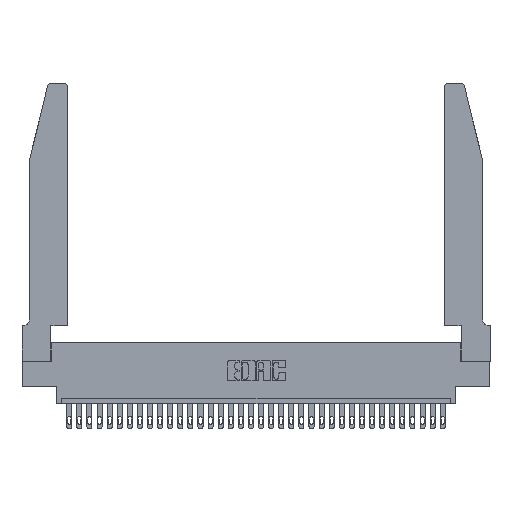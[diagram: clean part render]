
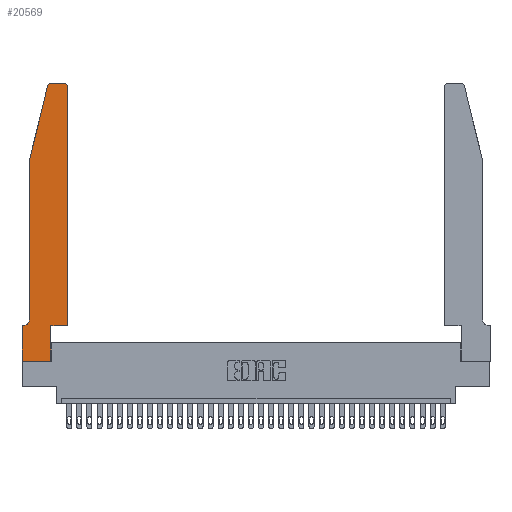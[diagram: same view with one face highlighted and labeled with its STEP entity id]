
A CAD part, top view. The second image highlights one B-rep face of the part: STEP entity #20569.
In plain terms, the highlighted planar face has unit normal (0, 0, 1).
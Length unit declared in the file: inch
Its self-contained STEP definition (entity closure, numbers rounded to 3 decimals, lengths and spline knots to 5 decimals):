
#305 = EDGE_CURVE ( 'NONE', #24303, #15757, #10780, .T. ) ;
#506 = CARTESIAN_POINT ( 'NONE',  ( 0.284, 2.72, 0.37 ) ) ;
#905 = CARTESIAN_POINT ( 'NONE',  ( 0.284, 2.75, 0.37 ) ) ;
#1224 = DIRECTION ( 'NONE',  ( 0., -1., 0. ) ) ;
#1340 = DIRECTION ( 'NONE',  ( 0., 0., -1. ) ) ;
#1395 = CARTESIAN_POINT ( 'NONE',  ( 0.4505, 2.72, 0.37 ) ) ;
#1404 = EDGE_CURVE ( 'NONE', #18840, #24303, #11525, .T. ) ;
#1493 = DIRECTION ( 'NONE',  ( -1., 0., 0. ) ) ;
#2607 = CARTESIAN_POINT ( 'NONE',  ( 0.4505, 0.35, 0.37 ) ) ;
#3799 = CARTESIAN_POINT ( 'NONE',  ( 0.4505, 0.35, 0.37 ) ) ;
#4000 = AXIS2_PLACEMENT_3D ( 'NONE', #31389, #18379, #26298 ) ;
#4079 = CARTESIAN_POINT ( 'NONE',  ( 0.4205, 2.75, 0.37 ) ) ;
#4186 = VERTEX_POINT ( 'NONE', #13802 ) ;
#4364 = VECTOR ( 'NONE', #33023, 39.37008 ) ;
#4469 = DIRECTION ( 'NONE',  ( 0., 0., 1. ) ) ;
#4846 = ORIENTED_EDGE ( 'NONE', *, *, #305, .T. ) ;
#4898 = VERTEX_POINT ( 'NONE', #23173 ) ;
#6002 = LINE ( 'NONE', #12059, #4364 ) ;
#6209 = CARTESIAN_POINT ( 'NONE',  ( 0.0755, 2., 0.37 ) ) ;
#6503 = LINE ( 'NONE', #12912, #21293 ) ;
#6768 = AXIS2_PLACEMENT_3D ( 'NONE', #17892, #4469, #20534 ) ;
#7193 = ORIENTED_EDGE ( 'NONE', *, *, #22379, .T. ) ;
#7827 = CARTESIAN_POINT ( 'NONE',  ( 0.0755, 0.35, 0.37 ) ) ;
#7880 = VECTOR ( 'NONE', #12998, 39.37008 ) ;
#8034 = ORIENTED_EDGE ( 'NONE', *, *, #8875, .T. ) ;
#8471 = EDGE_CURVE ( 'NONE', #13320, #4898, #28889, .T. ) ;
#8622 = LINE ( 'NONE', #22801, #30417 ) ;
#8875 = EDGE_CURVE ( 'NONE', #31925, #20930, #32997, .T. ) ;
#9761 = CARTESIAN_POINT ( 'NONE',  ( 0.0755, 2., 0.37 ) ) ;
#10780 = LINE ( 'NONE', #9761, #28857 ) ;
#11525 = CIRCLE ( 'NONE', #24944, 0.03 ) ;
#11659 = EDGE_CURVE ( 'NONE', #16005, #18840, #8622, .T. ) ;
#12059 = CARTESIAN_POINT ( 'NONE',  ( 0., 0., 0.37 ) ) ;
#12116 = LINE ( 'NONE', #7827, #25252 ) ;
#12176 = ORIENTED_EDGE ( 'NONE', *, *, #8471, .T. ) ;
#12217 = CARTESIAN_POINT ( 'NONE',  ( 0.0755, 0.42, 0.37 ) ) ;
#12607 = PLANE ( 'NONE',  #6768 ) ;
#12912 = CARTESIAN_POINT ( 'NONE',  ( 0.0755, 2., 0.37 ) ) ;
#12998 = DIRECTION ( 'NONE',  ( 0., 1., 0. ) ) ;
#13320 = VERTEX_POINT ( 'NONE', #28864 ) ;
#13802 = CARTESIAN_POINT ( 'NONE',  ( 0.4505, 0.35, 0.37 ) ) ;
#14091 = VECTOR ( 'NONE', #20321, 39.37008 ) ;
#14521 = VECTOR ( 'NONE', #1224, 39.37008 ) ;
#14833 = LINE ( 'NONE', #3799, #16866 ) ;
#14865 = LINE ( 'NONE', #2607, #7880 ) ;
#14997 = CIRCLE ( 'NONE', #21307, 0.07 ) ;
#15329 = DIRECTION ( 'NONE',  ( 0., -1., 0. ) ) ;
#15757 = VERTEX_POINT ( 'NONE', #6209 ) ;
#16005 = VERTEX_POINT ( 'NONE', #4079 ) ;
#16279 = ORIENTED_EDGE ( 'NONE', *, *, #22177, .T. ) ;
#16815 = VERTEX_POINT ( 'NONE', #12217 ) ;
#16866 = VECTOR ( 'NONE', #29827, 39.37008 ) ;
#17140 = CARTESIAN_POINT ( 'NONE',  ( 0., 0., 0.37 ) ) ;
#17892 = CARTESIAN_POINT ( 'NONE',  ( 0., 0.35, 0.37 ) ) ;
#18133 = ORIENTED_EDGE ( 'NONE', *, *, #30949, .T. ) ;
#18219 = VERTEX_POINT ( 'NONE', #1395 ) ;
#18251 = ORIENTED_EDGE ( 'NONE', *, *, #11659, .T. ) ;
#18259 = CIRCLE ( 'NONE', #4000, 0.03 ) ;
#18379 = DIRECTION ( 'NONE',  ( 0., 0., 1. ) ) ;
#18840 = VERTEX_POINT ( 'NONE', #905 ) ;
#19017 = ORIENTED_EDGE ( 'NONE', *, *, #1404, .T. ) ;
#19186 = DIRECTION ( 'NONE',  ( -1., 0., 0. ) ) ;
#19715 = EDGE_CURVE ( 'NONE', #20930, #13320, #6002, .T. ) ;
#20290 = FACE_OUTER_BOUND ( 'NONE', #28917, .T. ) ;
#20321 = DIRECTION ( 'NONE',  ( 0., 1., 0. ) ) ;
#20534 = DIRECTION ( 'NONE',  ( 1., 0., 0. ) ) ;
#20569 = ADVANCED_FACE ( 'NONE', ( #20290 ), #12607, .T. ) ;
#20879 = ORIENTED_EDGE ( 'NONE', *, *, #32941, .T. ) ;
#20930 = VERTEX_POINT ( 'NONE', #17140 ) ;
#21264 = ORIENTED_EDGE ( 'NONE', *, *, #25139, .T. ) ;
#21293 = VECTOR ( 'NONE', #15329, 39.37008 ) ;
#21307 = AXIS2_PLACEMENT_3D ( 'NONE', #24576, #1340, #19186 ) ;
#21671 = CARTESIAN_POINT ( 'NONE',  ( 0.0055, 0.35, 0.37 ) ) ;
#22073 = EDGE_CURVE ( 'NONE', #16815, #33818, #14997, .T. ) ;
#22177 = EDGE_CURVE ( 'NONE', #33818, #31925, #12116, .T. ) ;
#22379 = EDGE_CURVE ( 'NONE', #18219, #16005, #18259, .T. ) ;
#22801 = CARTESIAN_POINT ( 'NONE',  ( 0.2605, 2.75, 0.37 ) ) ;
#22962 = CARTESIAN_POINT ( 'NONE',  ( 0.2865, 0.35, 0.37 ) ) ;
#23173 = CARTESIAN_POINT ( 'NONE',  ( 0.2865, 0.35, 0.37 ) ) ;
#24303 = VERTEX_POINT ( 'NONE', #32137 ) ;
#24576 = CARTESIAN_POINT ( 'NONE',  ( 0.0055, 0.42, 0.37 ) ) ;
#24686 = CARTESIAN_POINT ( 'NONE',  ( 0., 0., 0.37 ) ) ;
#24944 = AXIS2_PLACEMENT_3D ( 'NONE', #506, #31902, #31691 ) ;
#25139 = EDGE_CURVE ( 'NONE', #4898, #4186, #14833, .T. ) ;
#25252 = VECTOR ( 'NONE', #29623, 39.37008 ) ;
#26250 = ORIENTED_EDGE ( 'NONE', *, *, #19715, .T. ) ;
#26298 = DIRECTION ( 'NONE',  ( 1., 0., 0. ) ) ;
#26934 = CARTESIAN_POINT ( 'NONE',  ( 0., 0.35, 0.37 ) ) ;
#28857 = VECTOR ( 'NONE', #29032, 39.37008 ) ;
#28864 = CARTESIAN_POINT ( 'NONE',  ( 0.2865, 0., 0.37 ) ) ;
#28889 = LINE ( 'NONE', #22962, #14091 ) ;
#28917 = EDGE_LOOP ( 'NONE', ( #18251, #19017, #4846, #20879, #33751, #16279, #8034, #26250, #12176, #21264, #18133, #7193 ) ) ;
#29032 = DIRECTION ( 'NONE',  ( -0.239, -0.971, 0. ) ) ;
#29623 = DIRECTION ( 'NONE',  ( -1., 0., 0. ) ) ;
#29827 = DIRECTION ( 'NONE',  ( 1., 0., 0. ) ) ;
#30417 = VECTOR ( 'NONE', #1493, 39.37008 ) ;
#30949 = EDGE_CURVE ( 'NONE', #4186, #18219, #14865, .T. ) ;
#31389 = CARTESIAN_POINT ( 'NONE',  ( 0.4205, 2.72, 0.37 ) ) ;
#31691 = DIRECTION ( 'NONE',  ( 1., 0., 0. ) ) ;
#31902 = DIRECTION ( 'NONE',  ( 0., 0., 1. ) ) ;
#31925 = VERTEX_POINT ( 'NONE', #26934 ) ;
#32137 = CARTESIAN_POINT ( 'NONE',  ( 0.25487, 2.72718, 0.37 ) ) ;
#32941 = EDGE_CURVE ( 'NONE', #15757, #16815, #6503, .T. ) ;
#32997 = LINE ( 'NONE', #24686, #14521 ) ;
#33023 = DIRECTION ( 'NONE',  ( 1., 0., 0. ) ) ;
#33751 = ORIENTED_EDGE ( 'NONE', *, *, #22073, .T. ) ;
#33818 = VERTEX_POINT ( 'NONE', #21671 ) ;
